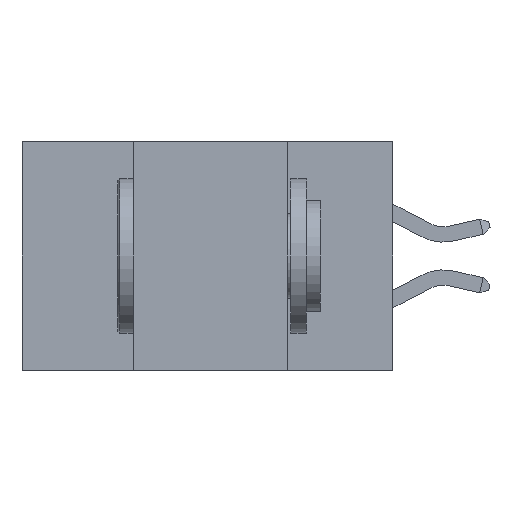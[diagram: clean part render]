
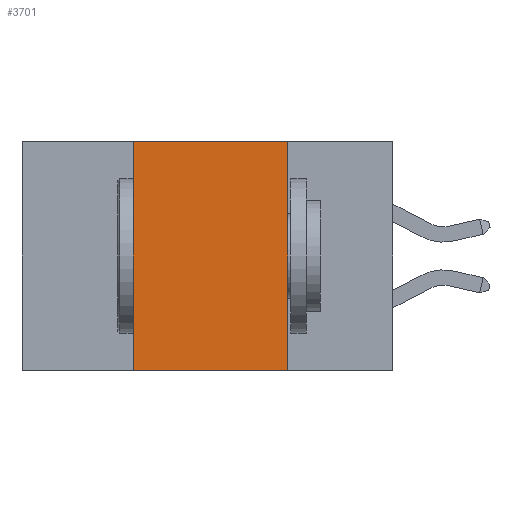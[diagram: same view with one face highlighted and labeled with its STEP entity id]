
A CAD part, left-side view. The second image highlights one B-rep face of the part: STEP entity #3701.
In plain terms, the highlighted planar face has unit normal (-1, 0, 0).
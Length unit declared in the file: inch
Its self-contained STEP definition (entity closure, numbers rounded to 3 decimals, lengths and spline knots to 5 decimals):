
#289 = PLANE ( 'NONE',  #13520 ) ;
#2003 = VECTOR ( 'NONE', #5267, 39.37008 ) ;
#2627 = ORIENTED_EDGE ( 'NONE', *, *, #8143, .F. ) ;
#2644 = EDGE_CURVE ( 'NONE', #12120, #18752, #22040, .T. ) ;
#2817 = CARTESIAN_POINT ( 'NONE',  ( 0., 0.6, -0.37 ) ) ;
#3270 = VECTOR ( 'NONE', #10526, 39.37008 ) ;
#3701 = ADVANCED_FACE ( 'NONE', ( #15803 ), #289, .F. ) ;
#4351 = CARTESIAN_POINT ( 'NONE',  ( 0., 0.42, 0. ) ) ;
#4660 = CARTESIAN_POINT ( 'NONE',  ( 0., 0.17, 0. ) ) ;
#5267 = DIRECTION ( 'NONE',  ( 0., -1., 0. ) ) ;
#5311 = DIRECTION ( 'NONE',  ( 0., 0., -1. ) ) ;
#7153 = CARTESIAN_POINT ( 'NONE',  ( 0., 0.6, 0. ) ) ;
#7495 = VECTOR ( 'NONE', #8961, 39.37008 ) ;
#8143 = EDGE_CURVE ( 'NONE', #19004, #10434, #18038, .T. ) ;
#8845 = CARTESIAN_POINT ( 'NONE',  ( 0., 0.6, 0. ) ) ;
#8961 = DIRECTION ( 'NONE',  ( 0., 0., -1. ) ) ;
#9811 = LINE ( 'NONE', #8845, #2003 ) ;
#10149 = ORIENTED_EDGE ( 'NONE', *, *, #17689, .F. ) ;
#10434 = VERTEX_POINT ( 'NONE', #4351 ) ;
#10526 = DIRECTION ( 'NONE',  ( 0., 0., 1. ) ) ;
#11131 = LINE ( 'NONE', #2817, #17051 ) ;
#12120 = VERTEX_POINT ( 'NONE', #4660 ) ;
#13292 = CARTESIAN_POINT ( 'NONE',  ( 0., 0.42, -0.37 ) ) ;
#13520 = AXIS2_PLACEMENT_3D ( 'NONE', #7153, #15840, #5311 ) ;
#13707 = ORIENTED_EDGE ( 'NONE', *, *, #2644, .F. ) ;
#14590 = CARTESIAN_POINT ( 'NONE',  ( 0., 0.17, -0.37 ) ) ;
#14708 = ORIENTED_EDGE ( 'NONE', *, *, #18085, .T. ) ;
#15622 = CARTESIAN_POINT ( 'NONE',  ( 0., 0.17, 0. ) ) ;
#15803 = FACE_OUTER_BOUND ( 'NONE', #22277, .T. ) ;
#15840 = DIRECTION ( 'NONE',  ( 1., 0., 0. ) ) ;
#16855 = CARTESIAN_POINT ( 'NONE',  ( 0., 0.42, 0. ) ) ;
#17051 = VECTOR ( 'NONE', #21874, 39.37008 ) ;
#17689 = EDGE_CURVE ( 'NONE', #10434, #12120, #9811, .T. ) ;
#18038 = LINE ( 'NONE', #16855, #3270 ) ;
#18085 = EDGE_CURVE ( 'NONE', #19004, #18752, #11131, .T. ) ;
#18752 = VERTEX_POINT ( 'NONE', #14590 ) ;
#19004 = VERTEX_POINT ( 'NONE', #13292 ) ;
#21874 = DIRECTION ( 'NONE',  ( 0., -1., 0. ) ) ;
#22040 = LINE ( 'NONE', #15622, #7495 ) ;
#22277 = EDGE_LOOP ( 'NONE', ( #13707, #10149, #2627, #14708 ) ) ;
